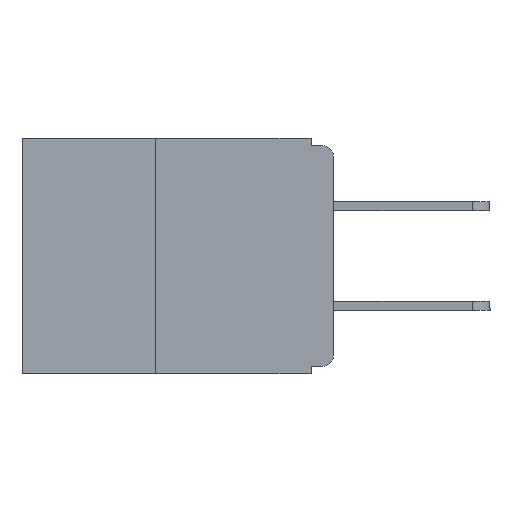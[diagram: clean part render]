
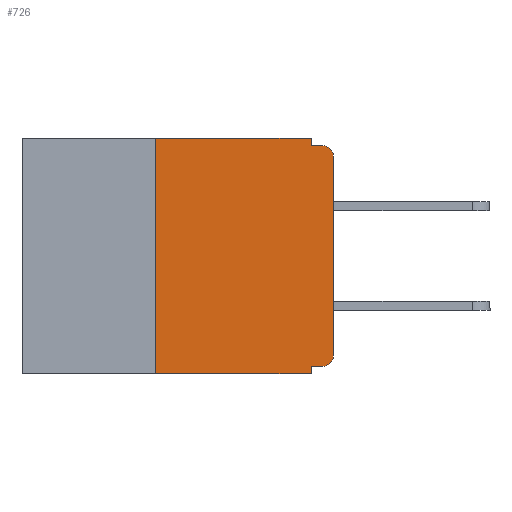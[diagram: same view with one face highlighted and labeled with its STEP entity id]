
A CAD part, left-side view. The second image highlights one B-rep face of the part: STEP entity #726.
In plain terms, the highlighted planar face has unit normal (-1, 0, 0).
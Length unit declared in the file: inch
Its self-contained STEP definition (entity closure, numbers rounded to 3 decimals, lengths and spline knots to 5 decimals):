
#241 = VECTOR ( 'NONE', #10183, 39.37008 ) ;
#249 = CARTESIAN_POINT ( 'NONE',  ( 0., 0.031, -0.33 ) ) ;
#323 = VECTOR ( 'NONE', #17218, 39.37008 ) ;
#706 = AXIS2_PLACEMENT_3D ( 'NONE', #10891, #11007, #14103 ) ;
#726 = ADVANCED_FACE ( 'NONE', ( #13357 ), #14139, .F. ) ;
#1586 = DIRECTION ( 'NONE',  ( 0., -1., 0. ) ) ;
#1790 = LINE ( 'NONE', #4358, #6944 ) ;
#1950 = EDGE_LOOP ( 'NONE', ( #3223, #1994, #3956, #12517, #7463, #4566, #3023, #5688, #12577, #2510 ) ) ;
#1994 = ORIENTED_EDGE ( 'NONE', *, *, #4863, .T. ) ;
#2218 = AXIS2_PLACEMENT_3D ( 'NONE', #13420, #4063, #14888 ) ;
#2510 = ORIENTED_EDGE ( 'NONE', *, *, #10881, .T. ) ;
#2536 = DIRECTION ( 'NONE',  ( 0., -1., 0. ) ) ;
#2603 = CARTESIAN_POINT ( 'NONE',  ( 0., 0., -0.025 ) ) ;
#2650 = LINE ( 'NONE', #14275, #11042 ) ;
#3023 = ORIENTED_EDGE ( 'NONE', *, *, #5306, .T. ) ;
#3213 = EDGE_CURVE ( 'NONE', #14198, #4843, #19118, .T. ) ;
#3223 = ORIENTED_EDGE ( 'NONE', *, *, #3213, .T. ) ;
#3582 = EDGE_CURVE ( 'NONE', #12085, #15123, #8641, .T. ) ;
#3951 = CARTESIAN_POINT ( 'NONE',  ( 0., 0.25, 0. ) ) ;
#3956 = ORIENTED_EDGE ( 'NONE', *, *, #19511, .F. ) ;
#4063 = DIRECTION ( 'NONE',  ( -1., 0., 0. ) ) ;
#4358 = CARTESIAN_POINT ( 'NONE',  ( 0., 0.25, -0.33 ) ) ;
#4399 = VERTEX_POINT ( 'NONE', #19329 ) ;
#4566 = ORIENTED_EDGE ( 'NONE', *, *, #12547, .F. ) ;
#4595 = CARTESIAN_POINT ( 'NONE',  ( 0., 0.031, -0.33 ) ) ;
#4843 = VERTEX_POINT ( 'NONE', #2603 ) ;
#4863 = EDGE_CURVE ( 'NONE', #4843, #11095, #11061, .T. ) ;
#4945 = EDGE_CURVE ( 'NONE', #4399, #14105, #17060, .T. ) ;
#5306 = EDGE_CURVE ( 'NONE', #14473, #11111, #2650, .T. ) ;
#5597 = CARTESIAN_POINT ( 'NONE',  ( 0., 0., -0.01 ) ) ;
#5688 = ORIENTED_EDGE ( 'NONE', *, *, #12198, .F. ) ;
#6873 = AXIS2_PLACEMENT_3D ( 'NONE', #19419, #19282, #19209 ) ;
#6944 = VECTOR ( 'NONE', #13704, 39.37008 ) ;
#7120 = VECTOR ( 'NONE', #2536, 39.37008 ) ;
#7153 = VECTOR ( 'NONE', #14300, 39.37008 ) ;
#7463 = ORIENTED_EDGE ( 'NONE', *, *, #9827, .F. ) ;
#8641 = LINE ( 'NONE', #9992, #241 ) ;
#8724 = CARTESIAN_POINT ( 'NONE',  ( 0., 0.031, 0. ) ) ;
#9694 = CARTESIAN_POINT ( 'NONE',  ( 0., 0.25, -0.33 ) ) ;
#9827 = EDGE_CURVE ( 'NONE', #17528, #12085, #10800, .T. ) ;
#9992 = CARTESIAN_POINT ( 'NONE',  ( 0., 0.031, 0. ) ) ;
#10183 = DIRECTION ( 'NONE',  ( 0., 0., -1. ) ) ;
#10335 = CARTESIAN_POINT ( 'NONE',  ( 0., 0.031, -0.32 ) ) ;
#10800 = LINE ( 'NONE', #11013, #11274 ) ;
#10881 = EDGE_CURVE ( 'NONE', #4399, #14198, #16335, .T. ) ;
#10891 = CARTESIAN_POINT ( 'NONE',  ( 0., 0.437, 0. ) ) ;
#11007 = DIRECTION ( 'NONE',  ( 1., 0., 0. ) ) ;
#11013 = CARTESIAN_POINT ( 'NONE',  ( 0., 0.437, 0. ) ) ;
#11042 = VECTOR ( 'NONE', #14899, 39.37008 ) ;
#11061 = CIRCLE ( 'NONE', #6873, 0.015 ) ;
#11095 = VERTEX_POINT ( 'NONE', #18219 ) ;
#11111 = VERTEX_POINT ( 'NONE', #4595 ) ;
#11274 = VECTOR ( 'NONE', #1586, 39.37008 ) ;
#11320 = LINE ( 'NONE', #5597, #7120 ) ;
#12085 = VERTEX_POINT ( 'NONE', #8724 ) ;
#12198 = EDGE_CURVE ( 'NONE', #14105, #11111, #12843, .T. ) ;
#12517 = ORIENTED_EDGE ( 'NONE', *, *, #3582, .F. ) ;
#12547 = EDGE_CURVE ( 'NONE', #14473, #17528, #1790, .T. ) ;
#12577 = ORIENTED_EDGE ( 'NONE', *, *, #4945, .F. ) ;
#12843 = LINE ( 'NONE', #249, #323 ) ;
#13357 = FACE_OUTER_BOUND ( 'NONE', #1950, .T. ) ;
#13420 = CARTESIAN_POINT ( 'NONE',  ( 0., 0.015, -0.305 ) ) ;
#13704 = DIRECTION ( 'NONE',  ( 0., 0., 1. ) ) ;
#14103 = DIRECTION ( 'NONE',  ( 0., 0., -1. ) ) ;
#14105 = VERTEX_POINT ( 'NONE', #10335 ) ;
#14139 = PLANE ( 'NONE',  #706 ) ;
#14198 = VERTEX_POINT ( 'NONE', #16512 ) ;
#14275 = CARTESIAN_POINT ( 'NONE',  ( 0., 0.437, -0.33 ) ) ;
#14300 = DIRECTION ( 'NONE',  ( 0., 0., 1. ) ) ;
#14319 = CARTESIAN_POINT ( 'NONE',  ( 0., 0., 0. ) ) ;
#14473 = VERTEX_POINT ( 'NONE', #9694 ) ;
#14888 = DIRECTION ( 'NONE',  ( 0., 0., -1. ) ) ;
#14899 = DIRECTION ( 'NONE',  ( 0., -1., 0. ) ) ;
#15123 = VERTEX_POINT ( 'NONE', #19126 ) ;
#16335 = CIRCLE ( 'NONE', #2218, 0.015 ) ;
#16512 = CARTESIAN_POINT ( 'NONE',  ( 0., 0., -0.305 ) ) ;
#16616 = VECTOR ( 'NONE', #18644, 39.37008 ) ;
#17060 = LINE ( 'NONE', #18771, #16616 ) ;
#17218 = DIRECTION ( 'NONE',  ( 0., 0., -1. ) ) ;
#17528 = VERTEX_POINT ( 'NONE', #3951 ) ;
#18219 = CARTESIAN_POINT ( 'NONE',  ( 0., 0.015, -0.01 ) ) ;
#18644 = DIRECTION ( 'NONE',  ( 0., 1., 0. ) ) ;
#18771 = CARTESIAN_POINT ( 'NONE',  ( 0., 0., -0.32 ) ) ;
#19118 = LINE ( 'NONE', #14319, #7153 ) ;
#19126 = CARTESIAN_POINT ( 'NONE',  ( 0., 0.031, -0.01 ) ) ;
#19209 = DIRECTION ( 'NONE',  ( 0., 0., -1. ) ) ;
#19282 = DIRECTION ( 'NONE',  ( -1., 0., 0. ) ) ;
#19329 = CARTESIAN_POINT ( 'NONE',  ( 0., 0.015, -0.32 ) ) ;
#19419 = CARTESIAN_POINT ( 'NONE',  ( 0., 0.015, -0.025 ) ) ;
#19511 = EDGE_CURVE ( 'NONE', #15123, #11095, #11320, .T. ) ;
